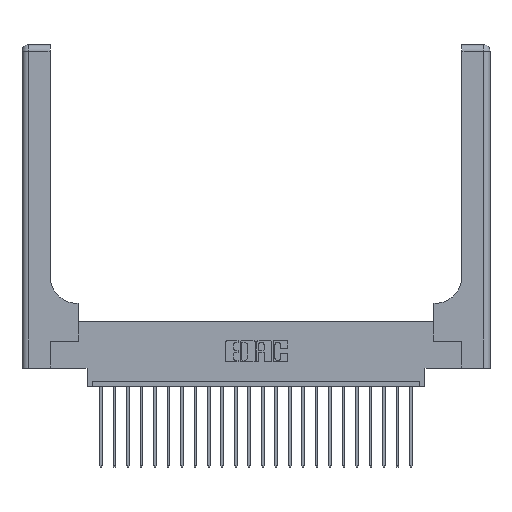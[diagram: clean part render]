
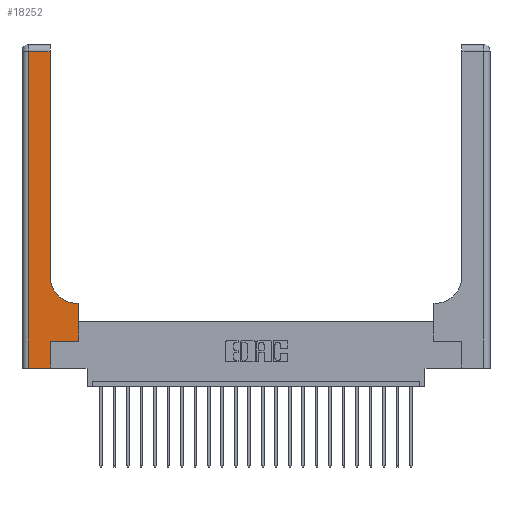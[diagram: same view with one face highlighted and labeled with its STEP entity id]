
A CAD part, top view. The second image highlights one B-rep face of the part: STEP entity #18252.
In plain terms, the highlighted planar face has unit normal (0, 0, 1).
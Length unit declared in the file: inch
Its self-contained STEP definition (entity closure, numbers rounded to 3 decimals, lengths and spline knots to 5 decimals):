
#478 = VERTEX_POINT ( 'NONE', #22656 ) ;
#498 = LINE ( 'NONE', #7646, #6757 ) ;
#901 = VERTEX_POINT ( 'NONE', #4856 ) ;
#1083 = EDGE_CURVE ( 'NONE', #901, #4998, #12592, .T. ) ;
#1451 = ORIENTED_EDGE ( 'NONE', *, *, #7293, .T. ) ;
#1858 = VERTEX_POINT ( 'NONE', #22286 ) ;
#2171 = DIRECTION ( 'NONE',  ( 0., 1., 0. ) ) ;
#2191 = CARTESIAN_POINT ( 'NONE',  ( 0., 2.94, 0.37 ) ) ;
#2665 = CARTESIAN_POINT ( 'NONE',  ( 0.06, 3., 0.37 ) ) ;
#2975 = CARTESIAN_POINT ( 'NONE',  ( 0.26, 0.6, 0.37 ) ) ;
#3563 = CARTESIAN_POINT ( 'NONE',  ( 0.51, 0.6, 0.37 ) ) ;
#3640 = CARTESIAN_POINT ( 'NONE',  ( 0.265, 0., 0.37 ) ) ;
#3711 = CARTESIAN_POINT ( 'NONE',  ( 0., 0., 0.37 ) ) ;
#3929 = CIRCLE ( 'NONE', #6945, 0.25 ) ;
#4101 = DIRECTION ( 'NONE',  ( 0., 1., 0. ) ) ;
#4501 = LINE ( 'NONE', #11657, #14498 ) ;
#4744 = ORIENTED_EDGE ( 'NONE', *, *, #19763, .T. ) ;
#4745 = ORIENTED_EDGE ( 'NONE', *, *, #17928, .T. ) ;
#4856 = CARTESIAN_POINT ( 'NONE',  ( 0.265, 0.25, 0.37 ) ) ;
#4998 = VERTEX_POINT ( 'NONE', #7553 ) ;
#5229 = CARTESIAN_POINT ( 'NONE',  ( 0., 3., 0.37 ) ) ;
#5470 = DIRECTION ( 'NONE',  ( -1., 0., 0. ) ) ;
#5481 = DIRECTION ( 'NONE',  ( 1., 0., 0. ) ) ;
#5946 = LINE ( 'NONE', #2191, #15485 ) ;
#5977 = LINE ( 'NONE', #13114, #18815 ) ;
#6057 = ORIENTED_EDGE ( 'NONE', *, *, #18752, .T. ) ;
#6757 = VECTOR ( 'NONE', #4101, 39.37008 ) ;
#6887 = VECTOR ( 'NONE', #14856, 39.37008 ) ;
#6945 = AXIS2_PLACEMENT_3D ( 'NONE', #11214, #21948, #16252 ) ;
#7293 = EDGE_CURVE ( 'NONE', #4998, #12177, #4501, .T. ) ;
#7536 = VECTOR ( 'NONE', #10127, 39.37008 ) ;
#7553 = CARTESIAN_POINT ( 'NONE',  ( 0.528, 0.25, 0.37 ) ) ;
#7565 = VERTEX_POINT ( 'NONE', #3563 ) ;
#7646 = CARTESIAN_POINT ( 'NONE',  ( 0.265, 0., 0.37 ) ) ;
#7953 = VERTEX_POINT ( 'NONE', #3640 ) ;
#8188 = EDGE_LOOP ( 'NONE', ( #6057, #19569, #4745, #9194, #11262, #17232, #1451, #12603, #4744 ) ) ;
#9194 = ORIENTED_EDGE ( 'NONE', *, *, #13137, .T. ) ;
#9345 = DIRECTION ( 'NONE',  ( -1., 0., 0. ) ) ;
#9413 = VECTOR ( 'NONE', #5481, 39.37008 ) ;
#9550 = CARTESIAN_POINT ( 'NONE',  ( 0.26, 0.85, 0.37 ) ) ;
#10127 = DIRECTION ( 'NONE',  ( -1., 0., 0. ) ) ;
#10722 = CARTESIAN_POINT ( 'NONE',  ( 0.265, 0.25, 0.37 ) ) ;
#11191 = EDGE_CURVE ( 'NONE', #7953, #901, #498, .T. ) ;
#11214 = CARTESIAN_POINT ( 'NONE',  ( 0.51, 0.85, 0.37 ) ) ;
#11262 = ORIENTED_EDGE ( 'NONE', *, *, #11191, .T. ) ;
#11657 = CARTESIAN_POINT ( 'NONE',  ( 0.528, 0.25, 0.37 ) ) ;
#12177 = VERTEX_POINT ( 'NONE', #16015 ) ;
#12373 = DIRECTION ( 'NONE',  ( 0., 0., -1. ) ) ;
#12592 = LINE ( 'NONE', #10722, #13513 ) ;
#12603 = ORIENTED_EDGE ( 'NONE', *, *, #15569, .T. ) ;
#12694 = DIRECTION ( 'NONE',  ( 1., 0., 0. ) ) ;
#13114 = CARTESIAN_POINT ( 'NONE',  ( 0.26, 3., 0.37 ) ) ;
#13137 = EDGE_CURVE ( 'NONE', #20743, #7953, #21488, .T. ) ;
#13513 = VECTOR ( 'NONE', #12694, 39.37008 ) ;
#13726 = VERTEX_POINT ( 'NONE', #9550 ) ;
#14498 = VECTOR ( 'NONE', #2171, 39.37008 ) ;
#14856 = DIRECTION ( 'NONE',  ( 0., -1., 0. ) ) ;
#15485 = VECTOR ( 'NONE', #9345, 39.37008 ) ;
#15569 = EDGE_CURVE ( 'NONE', #12177, #7565, #18993, .T. ) ;
#16015 = CARTESIAN_POINT ( 'NONE',  ( 0.528, 0.6, 0.37 ) ) ;
#16252 = DIRECTION ( 'NONE',  ( 1., 0., 0. ) ) ;
#16569 = AXIS2_PLACEMENT_3D ( 'NONE', #5229, #12373, #5470 ) ;
#17232 = ORIENTED_EDGE ( 'NONE', *, *, #1083, .T. ) ;
#17928 = EDGE_CURVE ( 'NONE', #1858, #20743, #18669, .T. ) ;
#18252 = ADVANCED_FACE ( 'NONE', ( #22999 ), #21242, .F. ) ;
#18669 = LINE ( 'NONE', #2665, #6887 ) ;
#18752 = EDGE_CURVE ( 'NONE', #13726, #478, #5977, .T. ) ;
#18815 = VECTOR ( 'NONE', #20245, 39.37008 ) ;
#18920 = EDGE_CURVE ( 'NONE', #478, #1858, #5946, .T. ) ;
#18993 = LINE ( 'NONE', #2975, #7536 ) ;
#19569 = ORIENTED_EDGE ( 'NONE', *, *, #18920, .T. ) ;
#19763 = EDGE_CURVE ( 'NONE', #7565, #13726, #3929, .T. ) ;
#19768 = CARTESIAN_POINT ( 'NONE',  ( 0.06, 0., 0.37 ) ) ;
#20245 = DIRECTION ( 'NONE',  ( 0., 1., 0. ) ) ;
#20743 = VERTEX_POINT ( 'NONE', #19768 ) ;
#21242 = PLANE ( 'NONE',  #16569 ) ;
#21488 = LINE ( 'NONE', #3711, #9413 ) ;
#21948 = DIRECTION ( 'NONE',  ( 0., 0., -1. ) ) ;
#22286 = CARTESIAN_POINT ( 'NONE',  ( 0.06, 2.94, 0.37 ) ) ;
#22656 = CARTESIAN_POINT ( 'NONE',  ( 0.26, 2.94, 0.37 ) ) ;
#22999 = FACE_OUTER_BOUND ( 'NONE', #8188, .T. ) ;
